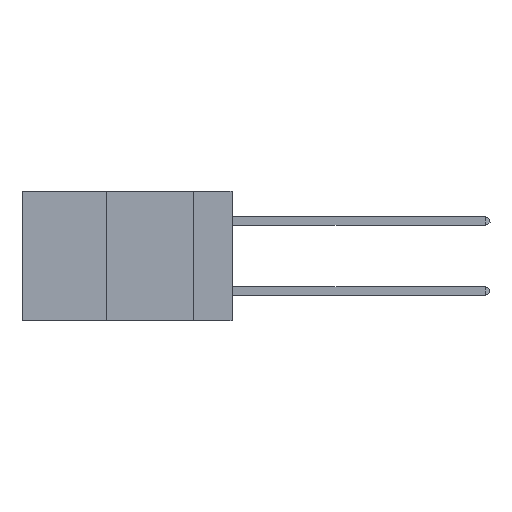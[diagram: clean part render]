
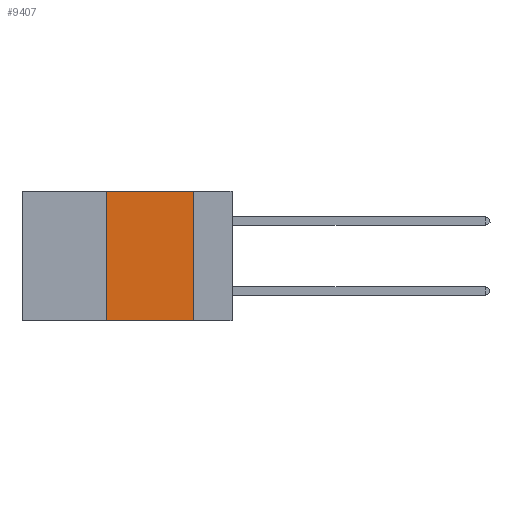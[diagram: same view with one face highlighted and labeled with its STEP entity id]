
A CAD part, left-side view. The second image highlights one B-rep face of the part: STEP entity #9407.
In plain terms, the highlighted planar face has unit normal (-1, 0, 0).
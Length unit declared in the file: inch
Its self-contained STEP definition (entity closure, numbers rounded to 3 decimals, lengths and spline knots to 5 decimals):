
#225 = VERTEX_POINT ( 'NONE', #12706 ) ;
#281 = VECTOR ( 'NONE', #8293, 39.37008 ) ;
#392 = DIRECTION ( 'NONE',  ( 0., -1., 0. ) ) ;
#681 = VERTEX_POINT ( 'NONE', #4603 ) ;
#1864 = CARTESIAN_POINT ( 'NONE',  ( 0., 0.11, 0. ) ) ;
#1888 = LINE ( 'NONE', #5974, #5933 ) ;
#2567 = LINE ( 'NONE', #9380, #281 ) ;
#2568 = PLANE ( 'NONE',  #7412 ) ;
#3109 = ORIENTED_EDGE ( 'NONE', *, *, #11033, .T. ) ;
#3370 = ORIENTED_EDGE ( 'NONE', *, *, #5136, .F. ) ;
#4124 = ORIENTED_EDGE ( 'NONE', *, *, #12280, .F. ) ;
#4598 = VECTOR ( 'NONE', #12933, 39.37008 ) ;
#4603 = CARTESIAN_POINT ( 'NONE',  ( 0., 0.36, -0.37 ) ) ;
#4798 = DIRECTION ( 'NONE',  ( 0., 0., -1. ) ) ;
#5136 = EDGE_CURVE ( 'NONE', #13661, #8158, #13052, .T. ) ;
#5933 = VECTOR ( 'NONE', #392, 39.37008 ) ;
#5974 = CARTESIAN_POINT ( 'NONE',  ( 0., 0.6, -0.37 ) ) ;
#5992 = CARTESIAN_POINT ( 'NONE',  ( 0., 0.6, 0. ) ) ;
#6046 = DIRECTION ( 'NONE',  ( 1., 0., 0. ) ) ;
#7112 = CARTESIAN_POINT ( 'NONE',  ( 0., 0.11, -0.37 ) ) ;
#7412 = AXIS2_PLACEMENT_3D ( 'NONE', #5992, #6046, #4798 ) ;
#8158 = VERTEX_POINT ( 'NONE', #7112 ) ;
#8293 = DIRECTION ( 'NONE',  ( 0., -1., 0. ) ) ;
#8751 = ORIENTED_EDGE ( 'NONE', *, *, #13997, .F. ) ;
#8940 = EDGE_LOOP ( 'NONE', ( #3370, #4124, #8751, #3109 ) ) ;
#9380 = CARTESIAN_POINT ( 'NONE',  ( 0., 0.6, 0. ) ) ;
#9407 = ADVANCED_FACE ( 'NONE', ( #14330 ), #2568, .F. ) ;
#9671 = DIRECTION ( 'NONE',  ( 0., 0., -1. ) ) ;
#9749 = LINE ( 'NONE', #11702, #4598 ) ;
#10404 = VECTOR ( 'NONE', #9671, 39.37008 ) ;
#10791 = CARTESIAN_POINT ( 'NONE',  ( 0., 0.11, 0. ) ) ;
#11033 = EDGE_CURVE ( 'NONE', #681, #8158, #1888, .T. ) ;
#11702 = CARTESIAN_POINT ( 'NONE',  ( 0., 0.36, 0. ) ) ;
#12280 = EDGE_CURVE ( 'NONE', #225, #13661, #2567, .T. ) ;
#12706 = CARTESIAN_POINT ( 'NONE',  ( 0., 0.36, 0. ) ) ;
#12933 = DIRECTION ( 'NONE',  ( 0., 0., 1. ) ) ;
#13052 = LINE ( 'NONE', #10791, #10404 ) ;
#13661 = VERTEX_POINT ( 'NONE', #1864 ) ;
#13997 = EDGE_CURVE ( 'NONE', #681, #225, #9749, .T. ) ;
#14330 = FACE_OUTER_BOUND ( 'NONE', #8940, .T. ) ;
